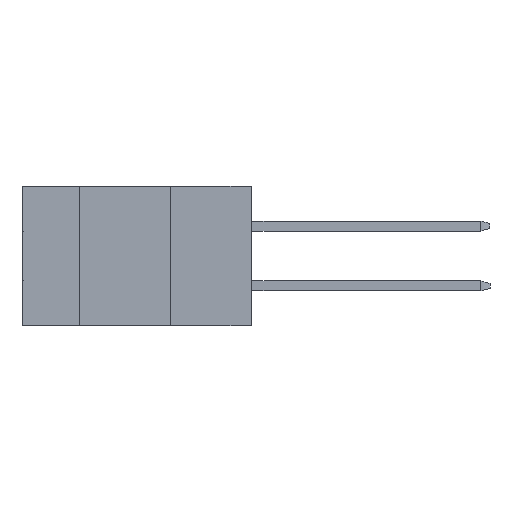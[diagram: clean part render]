
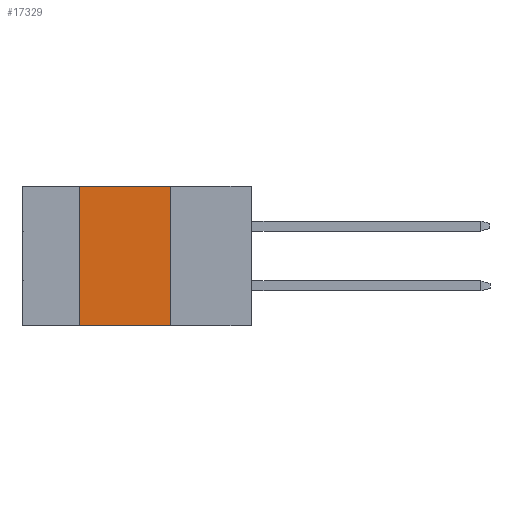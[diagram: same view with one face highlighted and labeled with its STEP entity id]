
A CAD part, left-side view. The second image highlights one B-rep face of the part: STEP entity #17329.
In plain terms, the highlighted planar face has unit normal (-1, 0, 0).
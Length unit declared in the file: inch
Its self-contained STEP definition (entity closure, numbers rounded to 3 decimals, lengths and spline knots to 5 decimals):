
#251 = LINE ( 'NONE', #20019, #15424 ) ;
#1989 = DIRECTION ( 'NONE',  ( 0., 0., -1. ) ) ;
#4150 = CARTESIAN_POINT ( 'NONE',  ( 0., 0.72, 0. ) ) ;
#4532 = DIRECTION ( 'NONE',  ( 0., 0., 1. ) ) ;
#4663 = LINE ( 'NONE', #17909, #19500 ) ;
#5690 = ORIENTED_EDGE ( 'NONE', *, *, #13255, .T. ) ;
#5907 = CARTESIAN_POINT ( 'NONE',  ( 0., 0.254, -0.437 ) ) ;
#6600 = DIRECTION ( 'NONE',  ( 0., -1., 0. ) ) ;
#6845 = VERTEX_POINT ( 'NONE', #16763 ) ;
#9098 = EDGE_LOOP ( 'NONE', ( #14187, #17082, #11007, #5690 ) ) ;
#9179 = VERTEX_POINT ( 'NONE', #5907 ) ;
#9243 = VERTEX_POINT ( 'NONE', #16581 ) ;
#9921 = EDGE_CURVE ( 'NONE', #13332, #9243, #14212, .T. ) ;
#10766 = DIRECTION ( 'NONE',  ( 1., 0., 0. ) ) ;
#11007 = ORIENTED_EDGE ( 'NONE', *, *, #9921, .F. ) ;
#11070 = LINE ( 'NONE', #20815, #11917 ) ;
#11917 = VECTOR ( 'NONE', #15761, 39.37008 ) ;
#12031 = EDGE_CURVE ( 'NONE', #9243, #6845, #4663, .T. ) ;
#13255 = EDGE_CURVE ( 'NONE', #13332, #9179, #11070, .T. ) ;
#13332 = VERTEX_POINT ( 'NONE', #15977 ) ;
#13752 = DIRECTION ( 'NONE',  ( 0., 0., -1. ) ) ;
#14076 = FACE_OUTER_BOUND ( 'NONE', #9098, .T. ) ;
#14187 = ORIENTED_EDGE ( 'NONE', *, *, #14257, .F. ) ;
#14212 = LINE ( 'NONE', #20777, #21206 ) ;
#14257 = EDGE_CURVE ( 'NONE', #6845, #9179, #251, .T. ) ;
#15424 = VECTOR ( 'NONE', #13752, 39.37008 ) ;
#15761 = DIRECTION ( 'NONE',  ( 0., -1., 0. ) ) ;
#15977 = CARTESIAN_POINT ( 'NONE',  ( 0., 0.54, -0.437 ) ) ;
#16581 = CARTESIAN_POINT ( 'NONE',  ( 0., 0.54, 0. ) ) ;
#16763 = CARTESIAN_POINT ( 'NONE',  ( 0., 0.254, 0. ) ) ;
#17082 = ORIENTED_EDGE ( 'NONE', *, *, #12031, .F. ) ;
#17329 = ADVANCED_FACE ( 'NONE', ( #14076 ), #20642, .F. ) ;
#17909 = CARTESIAN_POINT ( 'NONE',  ( 0., 0.72, 0. ) ) ;
#19500 = VECTOR ( 'NONE', #6600, 39.37008 ) ;
#20019 = CARTESIAN_POINT ( 'NONE',  ( 0., 0.254, -0.437 ) ) ;
#20468 = AXIS2_PLACEMENT_3D ( 'NONE', #4150, #10766, #1989 ) ;
#20642 = PLANE ( 'NONE',  #20468 ) ;
#20777 = CARTESIAN_POINT ( 'NONE',  ( 0., 0.54, -0.437 ) ) ;
#20815 = CARTESIAN_POINT ( 'NONE',  ( 0., 0.72, -0.437 ) ) ;
#21206 = VECTOR ( 'NONE', #4532, 39.37008 ) ;
